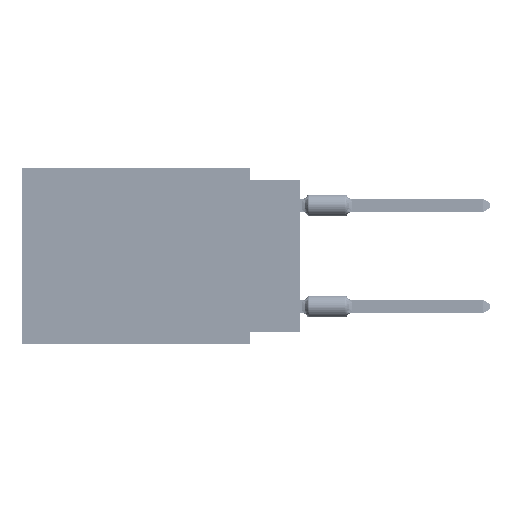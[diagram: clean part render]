
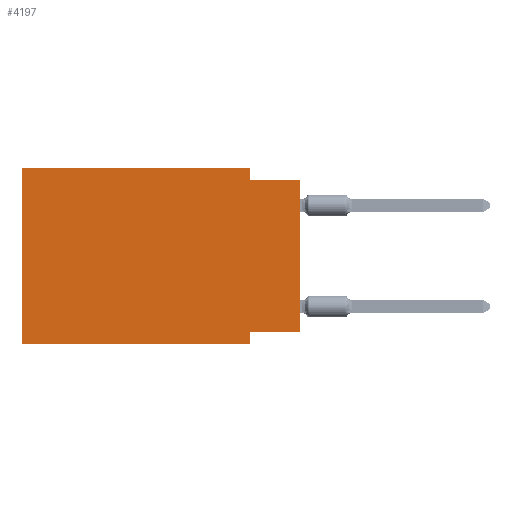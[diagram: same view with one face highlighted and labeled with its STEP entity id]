
A CAD part, left-side view. The second image highlights one B-rep face of the part: STEP entity #4197.
In plain terms, the highlighted planar face has unit normal (-1, 0, 0).
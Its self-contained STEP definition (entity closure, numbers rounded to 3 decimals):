
#1197 = AXIS2_PLACEMENT_3D ( 'NONE', #13202, #39239, #64879 ) ;
#1365 = EDGE_CURVE ( 'NONE', #38104, #28545, #6388, .T. ) ;
#1427 = ORIENTED_EDGE ( 'NONE', *, *, #27823, .F. ) ;
#4197 = ADVANCED_FACE ( 'NONE', ( #71161 ), #13602, .F. ) ;
#4316 = VECTOR ( 'NONE', #34313, 1000. ) ;
#5006 = LINE ( 'NONE', #6252, #5715 ) ;
#5715 = VECTOR ( 'NONE', #18851, 1000. ) ;
#6252 = CARTESIAN_POINT ( 'NONE',  ( 0., 0., -8.255 ) ) ;
#6388 = LINE ( 'NONE', #37074, #66366 ) ;
#6623 = ORIENTED_EDGE ( 'NONE', *, *, #34447, .F. ) ;
#9904 = CARTESIAN_POINT ( 'NONE',  ( 0., 13.97, -8.89 ) ) ;
#10043 = DIRECTION ( 'NONE',  ( 0., -1., 0. ) ) ;
#11826 = EDGE_CURVE ( 'NONE', #33145, #47693, #5006, .T. ) ;
#12197 = ORIENTED_EDGE ( 'NONE', *, *, #1365, .F. ) ;
#13096 = LINE ( 'NONE', #14339, #52023 ) ;
#13103 = DIRECTION ( 'NONE',  ( 0., 0., 1. ) ) ;
#13202 = CARTESIAN_POINT ( 'NONE',  ( 0., 13.97, 0. ) ) ;
#13203 = VERTEX_POINT ( 'NONE', #44928 ) ;
#13291 = EDGE_LOOP ( 'NONE', ( #74681, #1427, #38573, #6623, #12197, #59110, #63755, #56430 ) ) ;
#13602 = PLANE ( 'NONE',  #1197 ) ;
#14339 = CARTESIAN_POINT ( 'NONE',  ( 0., 13.97, -8.89 ) ) ;
#15258 = LINE ( 'NONE', #40073, #73760 ) ;
#15794 = CARTESIAN_POINT ( 'NONE',  ( 0., 2.54, -8.89 ) ) ;
#17996 = VECTOR ( 'NONE', #10043, 1000. ) ;
#18652 = CARTESIAN_POINT ( 'NONE',  ( 0., 2.54, -8.89 ) ) ;
#18851 = DIRECTION ( 'NONE',  ( 0., 1., 0. ) ) ;
#22852 = DIRECTION ( 'NONE',  ( 0., 0., 1. ) ) ;
#24181 = EDGE_CURVE ( 'NONE', #47693, #29212, #75365, .T. ) ;
#25877 = EDGE_CURVE ( 'NONE', #38104, #29212, #13096, .T. ) ;
#27823 = EDGE_CURVE ( 'NONE', #13203, #62332, #15258, .T. ) ;
#28545 = VERTEX_POINT ( 'NONE', #31907 ) ;
#29212 = VERTEX_POINT ( 'NONE', #15794 ) ;
#30176 = CARTESIAN_POINT ( 'NONE',  ( 0., 0., -8.255 ) ) ;
#31907 = CARTESIAN_POINT ( 'NONE',  ( 0., 13.97, 0. ) ) ;
#33145 = VERTEX_POINT ( 'NONE', #30176 ) ;
#34313 = DIRECTION ( 'NONE',  ( 0., 0., -1. ) ) ;
#34447 = EDGE_CURVE ( 'NONE', #28545, #69712, #48691, .T. ) ;
#36225 = VECTOR ( 'NONE', #22852, 1000. ) ;
#37074 = CARTESIAN_POINT ( 'NONE',  ( 0., 13.97, 0. ) ) ;
#37154 = DIRECTION ( 'NONE',  ( 0., 0., -1. ) ) ;
#38104 = VERTEX_POINT ( 'NONE', #9904 ) ;
#38573 = ORIENTED_EDGE ( 'NONE', *, *, #70768, .F. ) ;
#39239 = DIRECTION ( 'NONE',  ( 1., 0., 0. ) ) ;
#40073 = CARTESIAN_POINT ( 'NONE',  ( 0., 0., -0.635 ) ) ;
#42392 = CARTESIAN_POINT ( 'NONE',  ( 0., 13.97, 0. ) ) ;
#44824 = DIRECTION ( 'NONE',  ( 0., -1., 0. ) ) ;
#44928 = CARTESIAN_POINT ( 'NONE',  ( 0., 2.54, -0.635 ) ) ;
#45858 = DIRECTION ( 'NONE',  ( 0., -1., 0. ) ) ;
#47693 = VERTEX_POINT ( 'NONE', #76913 ) ;
#48691 = LINE ( 'NONE', #42392, #17996 ) ;
#51719 = CARTESIAN_POINT ( 'NONE',  ( 0., 2.54, 0. ) ) ;
#52023 = VECTOR ( 'NONE', #45858, 1000. ) ;
#56430 = ORIENTED_EDGE ( 'NONE', *, *, #11826, .F. ) ;
#59110 = ORIENTED_EDGE ( 'NONE', *, *, #25877, .T. ) ;
#62332 = VERTEX_POINT ( 'NONE', #66672 ) ;
#62918 = EDGE_CURVE ( 'NONE', #33145, #62332, #74113, .T. ) ;
#63755 = ORIENTED_EDGE ( 'NONE', *, *, #24181, .F. ) ;
#64879 = DIRECTION ( 'NONE',  ( 0., 0., -1. ) ) ;
#65017 = CARTESIAN_POINT ( 'NONE',  ( 0., 2.54, 0. ) ) ;
#66366 = VECTOR ( 'NONE', #13103, 1000. ) ;
#66672 = CARTESIAN_POINT ( 'NONE',  ( 0., 0., -0.635 ) ) ;
#69712 = VERTEX_POINT ( 'NONE', #51719 ) ;
#70768 = EDGE_CURVE ( 'NONE', #69712, #13203, #72137, .T. ) ;
#71161 = FACE_OUTER_BOUND ( 'NONE', #13291, .T. ) ;
#72137 = LINE ( 'NONE', #65017, #4316 ) ;
#73760 = VECTOR ( 'NONE', #44824, 1000. ) ;
#74113 = LINE ( 'NONE', #74524, #36225 ) ;
#74524 = CARTESIAN_POINT ( 'NONE',  ( 0., 0., 0. ) ) ;
#74681 = ORIENTED_EDGE ( 'NONE', *, *, #62918, .T. ) ;
#75365 = LINE ( 'NONE', #18652, #78637 ) ;
#76913 = CARTESIAN_POINT ( 'NONE',  ( 0., 2.54, -8.255 ) ) ;
#78637 = VECTOR ( 'NONE', #37154, 1000. ) ;
